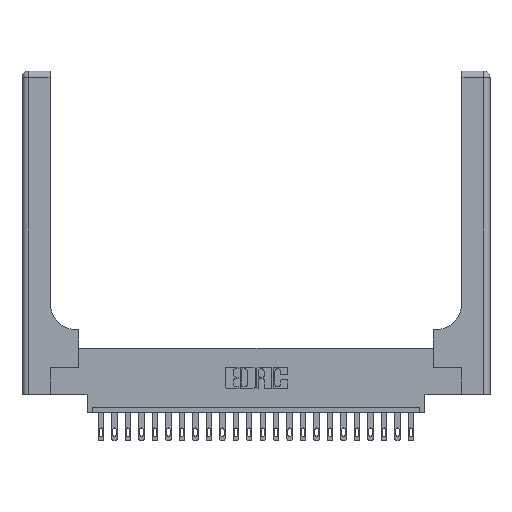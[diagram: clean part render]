
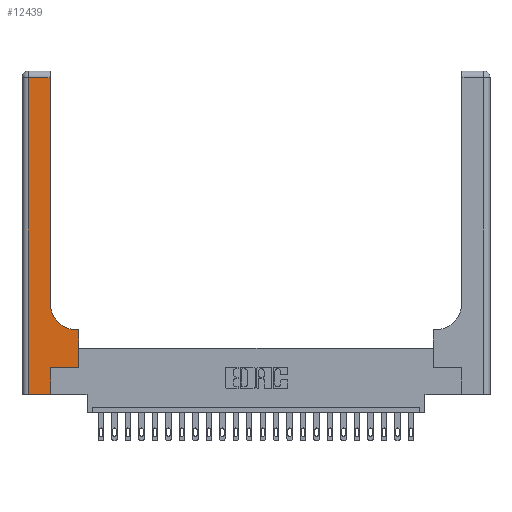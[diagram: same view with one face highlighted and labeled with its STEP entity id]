
A CAD part, top view. The second image highlights one B-rep face of the part: STEP entity #12439.
In plain terms, the highlighted planar face has unit normal (0, 0, 1).
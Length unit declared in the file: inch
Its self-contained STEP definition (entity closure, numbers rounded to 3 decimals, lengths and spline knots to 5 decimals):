
#221 = VERTEX_POINT ( 'NONE', #11501 ) ;
#235 = DIRECTION ( 'NONE',  ( 1., 0., 0. ) ) ;
#539 = CARTESIAN_POINT ( 'NONE',  ( 0., 3., 0.37 ) ) ;
#1095 = VERTEX_POINT ( 'NONE', #22186 ) ;
#2104 = CARTESIAN_POINT ( 'NONE',  ( 0.528, 0.6, 0.37 ) ) ;
#2310 = CARTESIAN_POINT ( 'NONE',  ( 0.26, 2.94, 0.37 ) ) ;
#2333 = VERTEX_POINT ( 'NONE', #22188 ) ;
#2724 = EDGE_CURVE ( 'NONE', #10858, #11360, #13100, .T. ) ;
#2996 = CARTESIAN_POINT ( 'NONE',  ( 0.265, 0., 0.37 ) ) ;
#3558 = ORIENTED_EDGE ( 'NONE', *, *, #2724, .T. ) ;
#3578 = EDGE_CURVE ( 'NONE', #22004, #3909, #4300, .T. ) ;
#3909 = VERTEX_POINT ( 'NONE', #7205 ) ;
#4024 = EDGE_CURVE ( 'NONE', #11360, #22004, #6449, .T. ) ;
#4300 = LINE ( 'NONE', #22109, #22532 ) ;
#4547 = VECTOR ( 'NONE', #9879, 39.37008 ) ;
#5416 = CARTESIAN_POINT ( 'NONE',  ( 0.26, 0.6, 0.37 ) ) ;
#5431 = VECTOR ( 'NONE', #19251, 39.37008 ) ;
#5696 = DIRECTION ( 'NONE',  ( 0., 1., 0. ) ) ;
#6123 = EDGE_CURVE ( 'NONE', #1095, #10858, #15894, .T. ) ;
#6153 = DIRECTION ( 'NONE',  ( 0., -1., 0. ) ) ;
#6449 = LINE ( 'NONE', #22743, #5431 ) ;
#7205 = CARTESIAN_POINT ( 'NONE',  ( 0.06, 0., 0.37 ) ) ;
#7511 = EDGE_CURVE ( 'NONE', #3909, #2333, #17321, .T. ) ;
#8129 = ORIENTED_EDGE ( 'NONE', *, *, #17684, .T. ) ;
#8463 = DIRECTION ( 'NONE',  ( -1., 0., 0. ) ) ;
#9157 = DIRECTION ( 'NONE',  ( -1., 0., 0. ) ) ;
#9486 = CARTESIAN_POINT ( 'NONE',  ( 0.26, 3., 0.37 ) ) ;
#9658 = DIRECTION ( 'NONE',  ( 0., 0., -1. ) ) ;
#9879 = DIRECTION ( 'NONE',  ( 0., 1., 0. ) ) ;
#9996 = CARTESIAN_POINT ( 'NONE',  ( 0.528, 0.25, 0.37 ) ) ;
#10481 = CARTESIAN_POINT ( 'NONE',  ( 0.06, 2.94, 0.37 ) ) ;
#10858 = VERTEX_POINT ( 'NONE', #13279 ) ;
#11360 = VERTEX_POINT ( 'NONE', #2310 ) ;
#11501 = CARTESIAN_POINT ( 'NONE',  ( 0.265, 0.25, 0.37 ) ) ;
#11637 = DIRECTION ( 'NONE',  ( 1., 0., 0. ) ) ;
#12236 = VECTOR ( 'NONE', #20295, 39.37008 ) ;
#12439 = ADVANCED_FACE ( 'NONE', ( #21717 ), #21610, .F. ) ;
#12482 = VECTOR ( 'NONE', #15055, 39.37008 ) ;
#12850 = VERTEX_POINT ( 'NONE', #2104 ) ;
#13100 = LINE ( 'NONE', #9486, #12482 ) ;
#13279 = CARTESIAN_POINT ( 'NONE',  ( 0.26, 0.85, 0.37 ) ) ;
#13996 = VECTOR ( 'NONE', #8463, 39.37008 ) ;
#14608 = EDGE_CURVE ( 'NONE', #2333, #221, #15104, .T. ) ;
#14933 = LINE ( 'NONE', #20187, #12236 ) ;
#15005 = LINE ( 'NONE', #21761, #22951 ) ;
#15055 = DIRECTION ( 'NONE',  ( 0., 1., 0. ) ) ;
#15104 = LINE ( 'NONE', #2996, #4547 ) ;
#15666 = LINE ( 'NONE', #5416, #13996 ) ;
#15894 = CIRCLE ( 'NONE', #17015, 0.25 ) ;
#16093 = ORIENTED_EDGE ( 'NONE', *, *, #14608, .T. ) ;
#16812 = AXIS2_PLACEMENT_3D ( 'NONE', #539, #17993, #9157 ) ;
#17012 = VECTOR ( 'NONE', #11637, 39.37008 ) ;
#17015 = AXIS2_PLACEMENT_3D ( 'NONE', #18139, #9658, #235 ) ;
#17321 = LINE ( 'NONE', #20478, #17012 ) ;
#17324 = ORIENTED_EDGE ( 'NONE', *, *, #7511, .T. ) ;
#17600 = ORIENTED_EDGE ( 'NONE', *, *, #4024, .T. ) ;
#17647 = ORIENTED_EDGE ( 'NONE', *, *, #3578, .T. ) ;
#17684 = EDGE_CURVE ( 'NONE', #20565, #12850, #15005, .T. ) ;
#17701 = ORIENTED_EDGE ( 'NONE', *, *, #6123, .T. ) ;
#17993 = DIRECTION ( 'NONE',  ( 0., 0., -1. ) ) ;
#18139 = CARTESIAN_POINT ( 'NONE',  ( 0.51, 0.85, 0.37 ) ) ;
#18496 = EDGE_CURVE ( 'NONE', #12850, #1095, #15666, .T. ) ;
#18703 = ORIENTED_EDGE ( 'NONE', *, *, #18496, .T. ) ;
#19251 = DIRECTION ( 'NONE',  ( -1., 0., 0. ) ) ;
#20187 = CARTESIAN_POINT ( 'NONE',  ( 0.265, 0.25, 0.37 ) ) ;
#20295 = DIRECTION ( 'NONE',  ( 1., 0., 0. ) ) ;
#20478 = CARTESIAN_POINT ( 'NONE',  ( 0., 0., 0.37 ) ) ;
#20565 = VERTEX_POINT ( 'NONE', #9996 ) ;
#20646 = ORIENTED_EDGE ( 'NONE', *, *, #21248, .T. ) ;
#21248 = EDGE_CURVE ( 'NONE', #221, #20565, #14933, .T. ) ;
#21610 = PLANE ( 'NONE',  #16812 ) ;
#21717 = FACE_OUTER_BOUND ( 'NONE', #22795, .T. ) ;
#21761 = CARTESIAN_POINT ( 'NONE',  ( 0.528, 0.25, 0.37 ) ) ;
#22004 = VERTEX_POINT ( 'NONE', #10481 ) ;
#22109 = CARTESIAN_POINT ( 'NONE',  ( 0.06, 3., 0.37 ) ) ;
#22186 = CARTESIAN_POINT ( 'NONE',  ( 0.51, 0.6, 0.37 ) ) ;
#22188 = CARTESIAN_POINT ( 'NONE',  ( 0.265, 0., 0.37 ) ) ;
#22532 = VECTOR ( 'NONE', #6153, 39.37008 ) ;
#22743 = CARTESIAN_POINT ( 'NONE',  ( 0., 2.94, 0.37 ) ) ;
#22795 = EDGE_LOOP ( 'NONE', ( #3558, #17600, #17647, #17324, #16093, #20646, #8129, #18703, #17701 ) ) ;
#22951 = VECTOR ( 'NONE', #5696, 39.37008 ) ;
